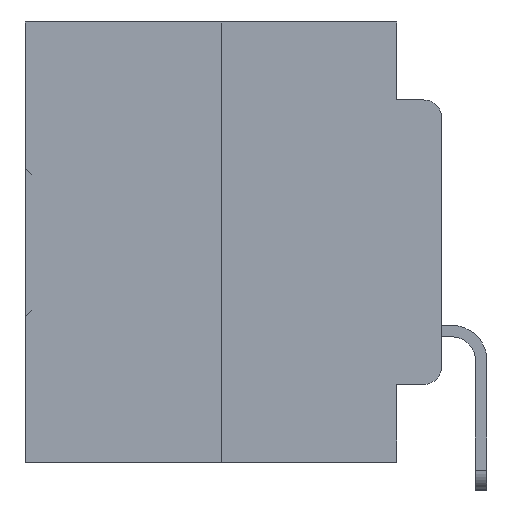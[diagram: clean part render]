
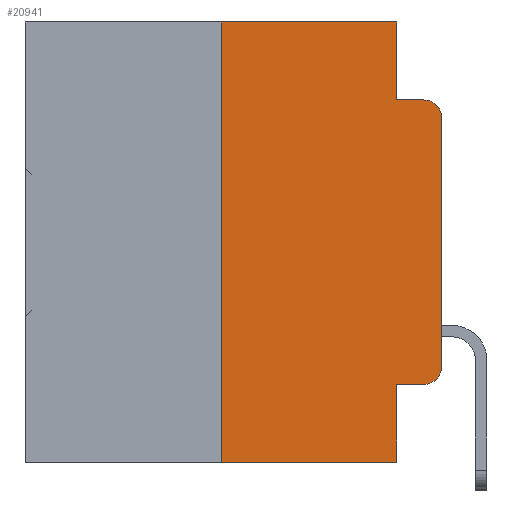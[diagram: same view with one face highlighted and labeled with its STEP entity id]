
A CAD part, left-side view. The second image highlights one B-rep face of the part: STEP entity #20941.
In plain terms, the highlighted planar face has unit normal (-1, 0, 0).
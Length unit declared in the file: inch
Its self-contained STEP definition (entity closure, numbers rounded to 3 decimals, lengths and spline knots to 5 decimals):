
#77 = EDGE_CURVE ( 'NONE', #25994, #19674, #19262, .T. ) ;
#581 = LINE ( 'NONE', #5013, #14717 ) ;
#828 = EDGE_CURVE ( 'NONE', #2042, #7176, #25412, .T. ) ;
#1418 = EDGE_LOOP ( 'NONE', ( #14316, #12232, #11557, #8944, #8513, #11702, #19421, #19655, #21866, #4130 ) ) ;
#1440 = CARTESIAN_POINT ( 'NONE',  ( 0., 0.051, 0. ) ) ;
#1785 = VECTOR ( 'NONE', #23082, 39.37008 ) ;
#1790 = VECTOR ( 'NONE', #6053, 39.37008 ) ;
#2042 = VERTEX_POINT ( 'NONE', #19882 ) ;
#2073 = DIRECTION ( 'NONE',  ( 0., 0., -1. ) ) ;
#2515 = DIRECTION ( 'NONE',  ( -1., 0., 0. ) ) ;
#3317 = VERTEX_POINT ( 'NONE', #21311 ) ;
#3350 = VERTEX_POINT ( 'NONE', #34561 ) ;
#3419 = LINE ( 'NONE', #4481, #32151 ) ;
#4130 = ORIENTED_EDGE ( 'NONE', *, *, #21882, .T. ) ;
#4360 = DIRECTION ( 'NONE',  ( 0., 0., -1. ) ) ;
#4481 = CARTESIAN_POINT ( 'NONE',  ( 0., 0.051, -0.4115 ) ) ;
#4793 = EDGE_CURVE ( 'NONE', #4942, #3317, #11862, .T. ) ;
#4942 = VERTEX_POINT ( 'NONE', #20573 ) ;
#5013 = CARTESIAN_POINT ( 'NONE',  ( 0., 0.473, -0.5 ) ) ;
#5482 = CARTESIAN_POINT ( 'NONE',  ( 0., 0.051, -0.0885 ) ) ;
#5571 = CARTESIAN_POINT ( 'NONE',  ( 0., 0.473, 0. ) ) ;
#6053 = DIRECTION ( 'NONE',  ( 0., 0., -1. ) ) ;
#7176 = VERTEX_POINT ( 'NONE', #25587 ) ;
#7274 = CARTESIAN_POINT ( 'NONE',  ( 0., 0.02, -0.0885 ) ) ;
#8153 = LINE ( 'NONE', #31722, #21610 ) ;
#8339 = DIRECTION ( 'NONE',  ( 0., -1., 0. ) ) ;
#8513 = ORIENTED_EDGE ( 'NONE', *, *, #25947, .F. ) ;
#8944 = ORIENTED_EDGE ( 'NONE', *, *, #19432, .F. ) ;
#9003 = VERTEX_POINT ( 'NONE', #26828 ) ;
#11194 = DIRECTION ( 'NONE',  ( 1., 0., 0. ) ) ;
#11557 = ORIENTED_EDGE ( 'NONE', *, *, #31835, .F. ) ;
#11702 = ORIENTED_EDGE ( 'NONE', *, *, #4793, .F. ) ;
#11862 = LINE ( 'NONE', #25022, #25184 ) ;
#12215 = LINE ( 'NONE', #5482, #32495 ) ;
#12232 = ORIENTED_EDGE ( 'NONE', *, *, #77, .T. ) ;
#13142 = VERTEX_POINT ( 'NONE', #32405 ) ;
#13217 = AXIS2_PLACEMENT_3D ( 'NONE', #19048, #2515, #21716 ) ;
#13455 = EDGE_CURVE ( 'NONE', #3350, #25994, #22831, .T. ) ;
#14316 = ORIENTED_EDGE ( 'NONE', *, *, #13455, .T. ) ;
#14717 = VECTOR ( 'NONE', #26673, 39.37008 ) ;
#15789 = LINE ( 'NONE', #24806, #1790 ) ;
#15888 = DIRECTION ( 'NONE',  ( 0., -1., 0. ) ) ;
#17087 = FACE_OUTER_BOUND ( 'NONE', #1418, .T. ) ;
#18155 = DIRECTION ( 'NONE',  ( 0., -1., 0. ) ) ;
#18354 = VECTOR ( 'NONE', #4360, 39.37008 ) ;
#18469 = AXIS2_PLACEMENT_3D ( 'NONE', #34342, #18649, #2073 ) ;
#18649 = DIRECTION ( 'NONE',  ( -1., 0., 0. ) ) ;
#19048 = CARTESIAN_POINT ( 'NONE',  ( 0., 0.02, -0.1085 ) ) ;
#19262 = CIRCLE ( 'NONE', #13217, 0.02 ) ;
#19421 = ORIENTED_EDGE ( 'NONE', *, *, #23922, .T. ) ;
#19432 = EDGE_CURVE ( 'NONE', #9003, #25280, #15789, .T. ) ;
#19655 = ORIENTED_EDGE ( 'NONE', *, *, #828, .F. ) ;
#19674 = VERTEX_POINT ( 'NONE', #7274 ) ;
#19882 = CARTESIAN_POINT ( 'NONE',  ( 0., 0.051, -0.4115 ) ) ;
#20573 = CARTESIAN_POINT ( 'NONE',  ( 0., 0.25, -0.5 ) ) ;
#20784 = CARTESIAN_POINT ( 'NONE',  ( 0., 0.051, -0.0885 ) ) ;
#20941 = ADVANCED_FACE ( 'NONE', ( #17087 ), #24480, .F. ) ;
#21311 = CARTESIAN_POINT ( 'NONE',  ( 0., 0.25, 0. ) ) ;
#21610 = VECTOR ( 'NONE', #15888, 39.37008 ) ;
#21716 = DIRECTION ( 'NONE',  ( 0., 0., -1. ) ) ;
#21866 = ORIENTED_EDGE ( 'NONE', *, *, #28996, .T. ) ;
#21882 = EDGE_CURVE ( 'NONE', #13142, #3350, #33863, .T. ) ;
#22831 = LINE ( 'NONE', #28407, #1785 ) ;
#23082 = DIRECTION ( 'NONE',  ( 0., 0., 1. ) ) ;
#23922 = EDGE_CURVE ( 'NONE', #4942, #7176, #581, .T. ) ;
#24480 = PLANE ( 'NONE',  #33415 ) ;
#24806 = CARTESIAN_POINT ( 'NONE',  ( 0., 0.051, 0. ) ) ;
#25022 = CARTESIAN_POINT ( 'NONE',  ( 0., 0.25, 0. ) ) ;
#25184 = VECTOR ( 'NONE', #27694, 39.37008 ) ;
#25280 = VERTEX_POINT ( 'NONE', #20784 ) ;
#25412 = LINE ( 'NONE', #1440, #18354 ) ;
#25587 = CARTESIAN_POINT ( 'NONE',  ( 0., 0.051, -0.5 ) ) ;
#25947 = EDGE_CURVE ( 'NONE', #3317, #9003, #8153, .T. ) ;
#25994 = VERTEX_POINT ( 'NONE', #26714 ) ;
#26673 = DIRECTION ( 'NONE',  ( 0., -1., 0. ) ) ;
#26714 = CARTESIAN_POINT ( 'NONE',  ( 0., 0., -0.1085 ) ) ;
#26828 = CARTESIAN_POINT ( 'NONE',  ( 0., 0.051, 0. ) ) ;
#27694 = DIRECTION ( 'NONE',  ( 0., 0., 1. ) ) ;
#28407 = CARTESIAN_POINT ( 'NONE',  ( 0., 0., 0. ) ) ;
#28996 = EDGE_CURVE ( 'NONE', #2042, #13142, #3419, .T. ) ;
#29786 = DIRECTION ( 'NONE',  ( 0., 0., -1. ) ) ;
#31722 = CARTESIAN_POINT ( 'NONE',  ( 0., 0.473, 0. ) ) ;
#31835 = EDGE_CURVE ( 'NONE', #25280, #19674, #12215, .T. ) ;
#32151 = VECTOR ( 'NONE', #18155, 39.37008 ) ;
#32405 = CARTESIAN_POINT ( 'NONE',  ( 0., 0.02, -0.4115 ) ) ;
#32495 = VECTOR ( 'NONE', #8339, 39.37008 ) ;
#33415 = AXIS2_PLACEMENT_3D ( 'NONE', #5571, #11194, #29786 ) ;
#33863 = CIRCLE ( 'NONE', #18469, 0.02 ) ;
#34342 = CARTESIAN_POINT ( 'NONE',  ( 0., 0.02, -0.3915 ) ) ;
#34561 = CARTESIAN_POINT ( 'NONE',  ( 0., 0., -0.3915 ) ) ;
